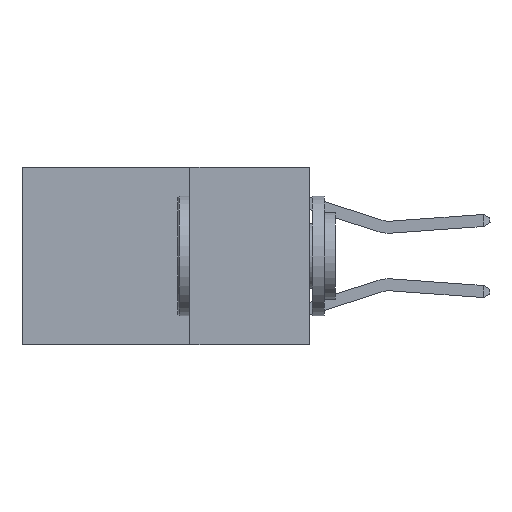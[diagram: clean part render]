
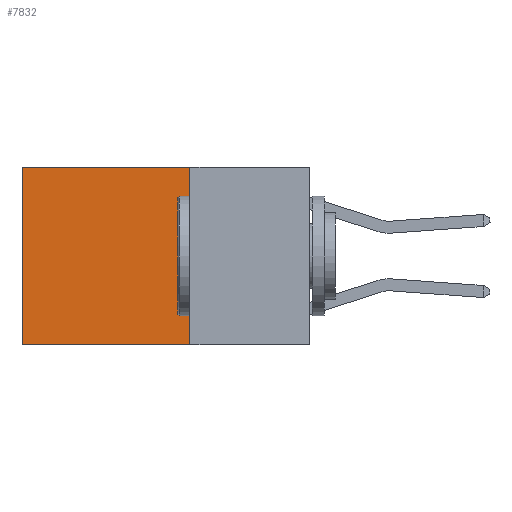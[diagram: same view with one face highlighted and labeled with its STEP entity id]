
A CAD part, left-side view. The second image highlights one B-rep face of the part: STEP entity #7832.
In plain terms, the highlighted planar face has unit normal (-1, 0, 0).
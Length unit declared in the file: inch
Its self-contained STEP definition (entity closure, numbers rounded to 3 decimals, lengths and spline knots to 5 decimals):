
#875 = EDGE_CURVE ( 'NONE', #8434, #11551, #1914, .T. ) ;
#1446 = DIRECTION ( 'NONE',  ( 0., 0., -1. ) ) ;
#1577 = CARTESIAN_POINT ( 'NONE',  ( 0.2625, 0.6, 0. ) ) ;
#1589 = VECTOR ( 'NONE', #8661, 39.37008 ) ;
#1648 = EDGE_LOOP ( 'NONE', ( #2134, #2404, #2485, #2719 ) ) ;
#1914 = LINE ( 'NONE', #2116, #9517 ) ;
#1918 = LINE ( 'NONE', #4805, #1589 ) ;
#2116 = CARTESIAN_POINT ( 'NONE',  ( 0.2625, 0.25, -0.37 ) ) ;
#2134 = ORIENTED_EDGE ( 'NONE', *, *, #8886, .T. ) ;
#2276 = DIRECTION ( 'NONE',  ( 0., 1., 0. ) ) ;
#2404 = ORIENTED_EDGE ( 'NONE', *, *, #875, .F. ) ;
#2485 = ORIENTED_EDGE ( 'NONE', *, *, #4377, .F. ) ;
#2633 = FACE_OUTER_BOUND ( 'NONE', #1648, .T. ) ;
#2719 = ORIENTED_EDGE ( 'NONE', *, *, #9954, .T. ) ;
#3394 = PLANE ( 'NONE',  #7043 ) ;
#3791 = DIRECTION ( 'NONE',  ( 0., 0., -1. ) ) ;
#4244 = LINE ( 'NONE', #9486, #11806 ) ;
#4377 = EDGE_CURVE ( 'NONE', #12516, #8434, #1918, .T. ) ;
#4805 = CARTESIAN_POINT ( 'NONE',  ( 0.2625, 0.25, 0. ) ) ;
#5186 = CARTESIAN_POINT ( 'NONE',  ( 0.2625, 0.25, -0.37 ) ) ;
#5324 = CARTESIAN_POINT ( 'NONE',  ( 0.2625, 0.25, 0. ) ) ;
#5796 = CARTESIAN_POINT ( 'NONE',  ( 0.2625, 0.25, 0. ) ) ;
#7043 = AXIS2_PLACEMENT_3D ( 'NONE', #5324, #7252, #1446 ) ;
#7252 = DIRECTION ( 'NONE',  ( 1., 0., 0. ) ) ;
#7832 = ADVANCED_FACE ( 'NONE', ( #2633 ), #3394, .F. ) ;
#8434 = VERTEX_POINT ( 'NONE', #5186 ) ;
#8661 = DIRECTION ( 'NONE',  ( 0., 0., -1. ) ) ;
#8665 = VERTEX_POINT ( 'NONE', #1577 ) ;
#8781 = DIRECTION ( 'NONE',  ( 0., 1., 0. ) ) ;
#8886 = EDGE_CURVE ( 'NONE', #8665, #11551, #4244, .T. ) ;
#9486 = CARTESIAN_POINT ( 'NONE',  ( 0.2625, 0.6, 0. ) ) ;
#9517 = VECTOR ( 'NONE', #8781, 39.37008 ) ;
#9540 = VECTOR ( 'NONE', #2276, 39.37008 ) ;
#9954 = EDGE_CURVE ( 'NONE', #12516, #8665, #12369, .T. ) ;
#11551 = VERTEX_POINT ( 'NONE', #12143 ) ;
#11696 = CARTESIAN_POINT ( 'NONE',  ( 0.2625, 0.25, 0. ) ) ;
#11806 = VECTOR ( 'NONE', #3791, 39.37008 ) ;
#12143 = CARTESIAN_POINT ( 'NONE',  ( 0.2625, 0.6, -0.37 ) ) ;
#12369 = LINE ( 'NONE', #11696, #9540 ) ;
#12516 = VERTEX_POINT ( 'NONE', #5796 ) ;
